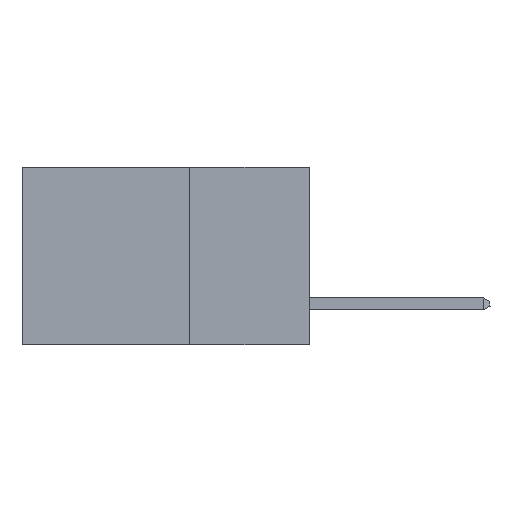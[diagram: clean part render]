
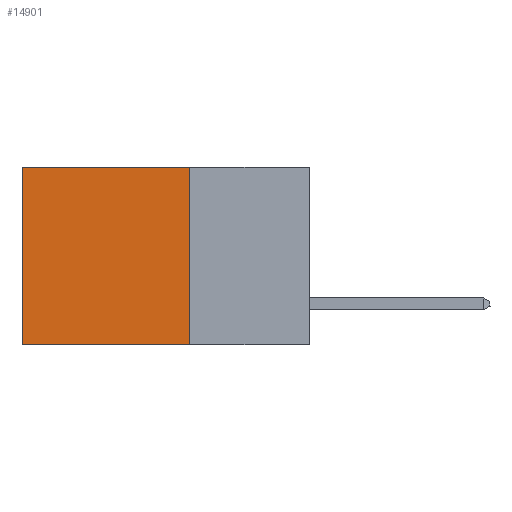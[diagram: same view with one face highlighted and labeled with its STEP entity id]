
A CAD part, left-side view. The second image highlights one B-rep face of the part: STEP entity #14901.
In plain terms, the highlighted planar face has unit normal (-1, 0, 0).
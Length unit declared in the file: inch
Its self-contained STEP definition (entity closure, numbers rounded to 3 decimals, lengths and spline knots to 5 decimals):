
#372 = DIRECTION ( 'NONE',  ( 0., 1., 0. ) ) ;
#994 = CARTESIAN_POINT ( 'NONE',  ( 0.2875, 0.25, 0. ) ) ;
#1089 = AXIS2_PLACEMENT_3D ( 'NONE', #994, #24333, #6934 ) ;
#1730 = EDGE_LOOP ( 'NONE', ( #7762, #18249, #24976, #33797 ) ) ;
#2142 = DIRECTION ( 'NONE',  ( 0., 0., -1. ) ) ;
#2292 = CARTESIAN_POINT ( 'NONE',  ( 0.2875, 0.6, 0. ) ) ;
#3156 = EDGE_CURVE ( 'NONE', #7367, #19683, #32881, .T. ) ;
#4338 = VERTEX_POINT ( 'NONE', #16794 ) ;
#4624 = EDGE_CURVE ( 'NONE', #4338, #7367, #23705, .T. ) ;
#6934 = DIRECTION ( 'NONE',  ( 0., 0., -1. ) ) ;
#7367 = VERTEX_POINT ( 'NONE', #33976 ) ;
#7762 = ORIENTED_EDGE ( 'NONE', *, *, #3156, .T. ) ;
#11025 = VECTOR ( 'NONE', #372, 39.37008 ) ;
#14901 = ADVANCED_FACE ( 'NONE', ( #36232 ), #27391, .F. ) ;
#16591 = CARTESIAN_POINT ( 'NONE',  ( 0.2875, 0.25, -0.37 ) ) ;
#16794 = CARTESIAN_POINT ( 'NONE',  ( 0.2875, 0.25, 0. ) ) ;
#17563 = CARTESIAN_POINT ( 'NONE',  ( 0.2875, 0.25, 0. ) ) ;
#18249 = ORIENTED_EDGE ( 'NONE', *, *, #34202, .F. ) ;
#18389 = CARTESIAN_POINT ( 'NONE',  ( 0.2875, 0.25, -0.37 ) ) ;
#18484 = LINE ( 'NONE', #17563, #27558 ) ;
#19683 = VERTEX_POINT ( 'NONE', #33246 ) ;
#20176 = VECTOR ( 'NONE', #2142, 39.37008 ) ;
#23705 = LINE ( 'NONE', #23959, #11025 ) ;
#23959 = CARTESIAN_POINT ( 'NONE',  ( 0.2875, 0.25, 0. ) ) ;
#24333 = DIRECTION ( 'NONE',  ( 1., 0., 0. ) ) ;
#24976 = ORIENTED_EDGE ( 'NONE', *, *, #26974, .F. ) ;
#25609 = DIRECTION ( 'NONE',  ( 0., 1., 0. ) ) ;
#25950 = DIRECTION ( 'NONE',  ( 0., 0., -1. ) ) ;
#26974 = EDGE_CURVE ( 'NONE', #4338, #35538, #18484, .T. ) ;
#26999 = LINE ( 'NONE', #16591, #27932 ) ;
#27391 = PLANE ( 'NONE',  #1089 ) ;
#27558 = VECTOR ( 'NONE', #25950, 39.37008 ) ;
#27932 = VECTOR ( 'NONE', #25609, 39.37008 ) ;
#32881 = LINE ( 'NONE', #2292, #20176 ) ;
#33246 = CARTESIAN_POINT ( 'NONE',  ( 0.2875, 0.6, -0.37 ) ) ;
#33797 = ORIENTED_EDGE ( 'NONE', *, *, #4624, .T. ) ;
#33976 = CARTESIAN_POINT ( 'NONE',  ( 0.2875, 0.6, 0. ) ) ;
#34202 = EDGE_CURVE ( 'NONE', #35538, #19683, #26999, .T. ) ;
#35538 = VERTEX_POINT ( 'NONE', #18389 ) ;
#36232 = FACE_OUTER_BOUND ( 'NONE', #1730, .T. ) ;
